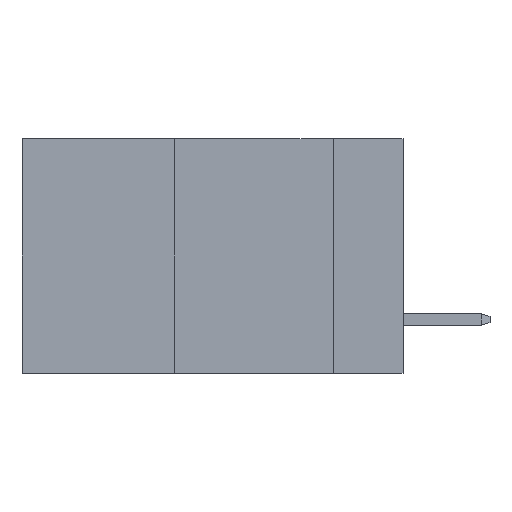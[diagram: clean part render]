
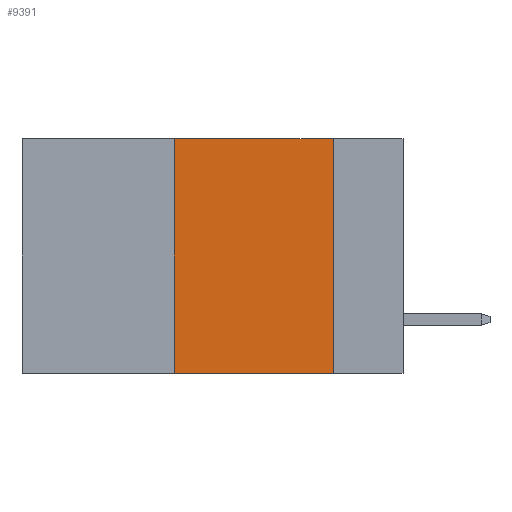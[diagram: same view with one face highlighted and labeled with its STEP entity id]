
A CAD part, left-side view. The second image highlights one B-rep face of the part: STEP entity #9391.
In plain terms, the highlighted planar face has unit normal (-1, 0, 0).
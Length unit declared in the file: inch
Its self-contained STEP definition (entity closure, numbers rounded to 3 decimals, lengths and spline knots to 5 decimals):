
#427 = EDGE_CURVE ( 'NONE', #9171, #1911, #5293, .T. ) ;
#542 = CARTESIAN_POINT ( 'NONE',  ( 0., 0.36, 0. ) ) ;
#1339 = DIRECTION ( 'NONE',  ( 0., -1., 0. ) ) ;
#1429 = CARTESIAN_POINT ( 'NONE',  ( 0., 0.11, 0. ) ) ;
#1506 = DIRECTION ( 'NONE',  ( 0., 0., 1. ) ) ;
#1765 = CARTESIAN_POINT ( 'NONE',  ( 0., 0.6, 0. ) ) ;
#1911 = VERTEX_POINT ( 'NONE', #4301 ) ;
#2127 = VECTOR ( 'NONE', #4548, 39.37008 ) ;
#2514 = VECTOR ( 'NONE', #1506, 39.37008 ) ;
#3013 = ORIENTED_EDGE ( 'NONE', *, *, #427, .F. ) ;
#3769 = ORIENTED_EDGE ( 'NONE', *, *, #7394, .F. ) ;
#3776 = CARTESIAN_POINT ( 'NONE',  ( 0., 0.6, 0. ) ) ;
#3995 = VECTOR ( 'NONE', #1339, 39.37008 ) ;
#4301 = CARTESIAN_POINT ( 'NONE',  ( 0., 0.11, -0.37 ) ) ;
#4548 = DIRECTION ( 'NONE',  ( 0., -1., 0. ) ) ;
#4647 = AXIS2_PLACEMENT_3D ( 'NONE', #1765, #10129, #11167 ) ;
#5025 = LINE ( 'NONE', #3776, #3995 ) ;
#5293 = LINE ( 'NONE', #1429, #7086 ) ;
#5596 = ORIENTED_EDGE ( 'NONE', *, *, #10833, .F. ) ;
#6288 = FACE_OUTER_BOUND ( 'NONE', #6449, .T. ) ;
#6358 = PLANE ( 'NONE',  #4647 ) ;
#6449 = EDGE_LOOP ( 'NONE', ( #3013, #3769, #5596, #10959 ) ) ;
#6715 = VERTEX_POINT ( 'NONE', #8290 ) ;
#7086 = VECTOR ( 'NONE', #10768, 39.37008 ) ;
#7219 = LINE ( 'NONE', #11187, #2127 ) ;
#7394 = EDGE_CURVE ( 'NONE', #9297, #9171, #5025, .T. ) ;
#7445 = CARTESIAN_POINT ( 'NONE',  ( 0., 0.36, 0. ) ) ;
#8008 = CARTESIAN_POINT ( 'NONE',  ( 0., 0.11, 0. ) ) ;
#8290 = CARTESIAN_POINT ( 'NONE',  ( 0., 0.36, -0.37 ) ) ;
#8883 = EDGE_CURVE ( 'NONE', #6715, #1911, #7219, .T. ) ;
#9171 = VERTEX_POINT ( 'NONE', #8008 ) ;
#9297 = VERTEX_POINT ( 'NONE', #7445 ) ;
#9391 = ADVANCED_FACE ( 'NONE', ( #6288 ), #6358, .F. ) ;
#10129 = DIRECTION ( 'NONE',  ( 1., 0., 0. ) ) ;
#10768 = DIRECTION ( 'NONE',  ( 0., 0., -1. ) ) ;
#10796 = LINE ( 'NONE', #542, #2514 ) ;
#10833 = EDGE_CURVE ( 'NONE', #6715, #9297, #10796, .T. ) ;
#10959 = ORIENTED_EDGE ( 'NONE', *, *, #8883, .T. ) ;
#11167 = DIRECTION ( 'NONE',  ( 0., 0., -1. ) ) ;
#11187 = CARTESIAN_POINT ( 'NONE',  ( 0., 0.6, -0.37 ) ) ;
